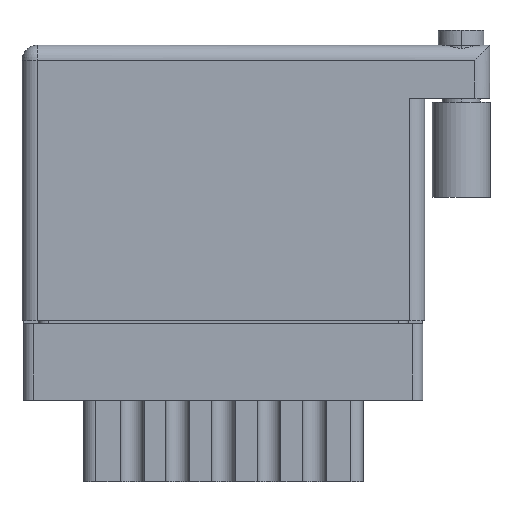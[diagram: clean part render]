
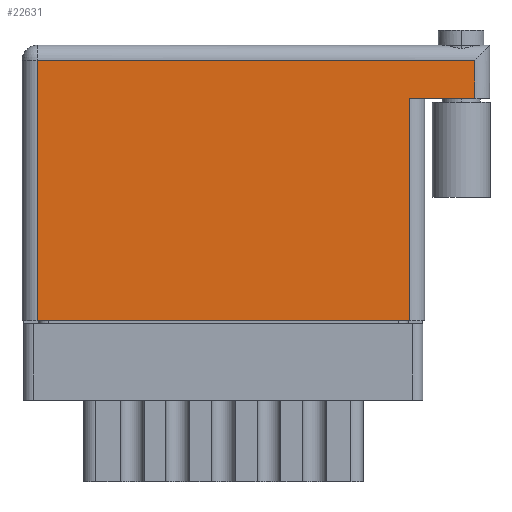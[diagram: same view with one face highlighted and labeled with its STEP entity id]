
A CAD part, front view. The second image highlights one B-rep face of the part: STEP entity #22631.
In plain terms, the highlighted face is planar.
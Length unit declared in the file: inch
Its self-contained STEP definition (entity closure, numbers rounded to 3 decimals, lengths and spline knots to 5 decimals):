
#24 = CARTESIAN_POINT ( 'NONE',  ( 0.05, 0., 0. ) ) ;
#1682 = DIRECTION ( 'NONE',  ( 0., 1., 0. ) ) ;
#1788 = LINE ( 'NONE', #4219, #9424 ) ;
#1816 = DIRECTION ( 'NONE',  ( -1., 0., 0. ) ) ;
#2972 = VERTEX_POINT ( 'NONE', #22951 ) ;
#3617 = CARTESIAN_POINT ( 'NONE',  ( 1.275, 0.731, 0. ) ) ;
#4219 = CARTESIAN_POINT ( 'NONE',  ( 0., 0., 0. ) ) ;
#4314 = VECTOR ( 'NONE', #6080, 39.37008 ) ;
#5351 = CARTESIAN_POINT ( 'NONE',  ( 1.489, 0.906, 0. ) ) ;
#5514 = VERTEX_POINT ( 'NONE', #14209 ) ;
#5779 = VECTOR ( 'NONE', #15590, 39.37008 ) ;
#5810 = DIRECTION ( 'NONE',  ( 0., 0., -1. ) ) ;
#6029 = EDGE_CURVE ( 'NONE', #19046, #9898, #1788, .T. ) ;
#6080 = DIRECTION ( 'NONE',  ( -1., 0., 0. ) ) ;
#6428 = CARTESIAN_POINT ( 'NONE',  ( 0.05, 0.856, 0. ) ) ;
#7584 = ORIENTED_EDGE ( 'NONE', *, *, #12221, .T. ) ;
#8801 = LINE ( 'NONE', #3617, #18597 ) ;
#9424 = VECTOR ( 'NONE', #14457, 39.37008 ) ;
#9587 = LINE ( 'NONE', #17652, #5779 ) ;
#9795 = CARTESIAN_POINT ( 'NONE',  ( 0., 0.906, 0. ) ) ;
#9898 = VERTEX_POINT ( 'NONE', #24789 ) ;
#10439 = ORIENTED_EDGE ( 'NONE', *, *, #16005, .T. ) ;
#10502 = VERTEX_POINT ( 'NONE', #15420 ) ;
#10719 = DIRECTION ( 'NONE',  ( -1., 0., 0. ) ) ;
#10763 = EDGE_LOOP ( 'NONE', ( #22439, #7584, #22757, #10439, #20457, #15464 ) ) ;
#12047 = LINE ( 'NONE', #5351, #23452 ) ;
#12086 = AXIS2_PLACEMENT_3D ( 'NONE', #9795, #5810, #1816 ) ;
#12221 = EDGE_CURVE ( 'NONE', #9898, #2972, #8801, .T. ) ;
#13901 = PLANE ( 'NONE',  #12086 ) ;
#14209 = CARTESIAN_POINT ( 'NONE',  ( 1.489, 0.731, 0. ) ) ;
#14457 = DIRECTION ( 'NONE',  ( 1., 0., 0. ) ) ;
#15283 = EDGE_CURVE ( 'NONE', #19151, #19046, #9587, .T. ) ;
#15420 = CARTESIAN_POINT ( 'NONE',  ( 1.489, 0.856, 0. ) ) ;
#15464 = ORIENTED_EDGE ( 'NONE', *, *, #15283, .T. ) ;
#15590 = DIRECTION ( 'NONE',  ( 0., -1., 0. ) ) ;
#16005 = EDGE_CURVE ( 'NONE', #5514, #10502, #12047, .T. ) ;
#16883 = FACE_OUTER_BOUND ( 'NONE', #10763, .T. ) ;
#17652 = CARTESIAN_POINT ( 'NONE',  ( 0.05, 0., 0. ) ) ;
#18158 = CARTESIAN_POINT ( 'NONE',  ( 1.539, 0.731, 0. ) ) ;
#18174 = EDGE_CURVE ( 'NONE', #10502, #19151, #25215, .T. ) ;
#18254 = VECTOR ( 'NONE', #10719, 39.37008 ) ;
#18597 = VECTOR ( 'NONE', #1682, 39.37008 ) ;
#19046 = VERTEX_POINT ( 'NONE', #24 ) ;
#19151 = VERTEX_POINT ( 'NONE', #6428 ) ;
#19481 = DIRECTION ( 'NONE',  ( 0., 1., 0. ) ) ;
#20457 = ORIENTED_EDGE ( 'NONE', *, *, #18174, .T. ) ;
#20681 = EDGE_CURVE ( 'NONE', #5514, #2972, #25880, .T. ) ;
#22439 = ORIENTED_EDGE ( 'NONE', *, *, #6029, .T. ) ;
#22631 = ADVANCED_FACE ( 'NONE', ( #16883 ), #13901, .F. ) ;
#22757 = ORIENTED_EDGE ( 'NONE', *, *, #20681, .F. ) ;
#22951 = CARTESIAN_POINT ( 'NONE',  ( 1.275, 0.731, 0. ) ) ;
#23452 = VECTOR ( 'NONE', #19481, 39.37008 ) ;
#24789 = CARTESIAN_POINT ( 'NONE',  ( 1.275, 0., 0. ) ) ;
#25206 = CARTESIAN_POINT ( 'NONE',  ( 0., 0.856, 0. ) ) ;
#25215 = LINE ( 'NONE', #25206, #18254 ) ;
#25880 = LINE ( 'NONE', #18158, #4314 ) ;
